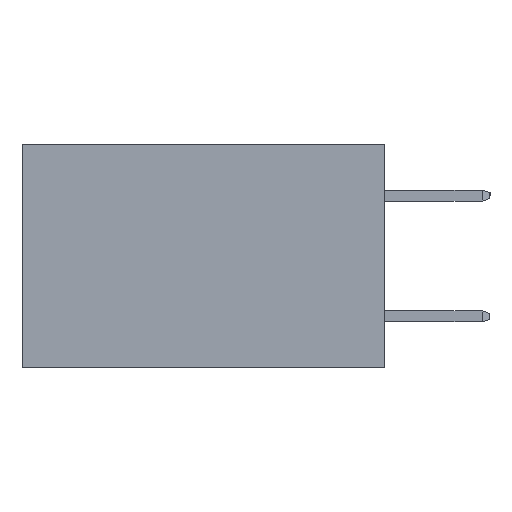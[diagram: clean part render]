
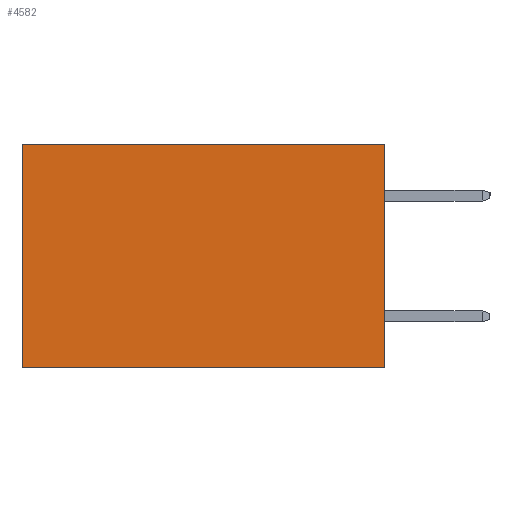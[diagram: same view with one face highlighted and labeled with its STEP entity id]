
A CAD part, left-side view. The second image highlights one B-rep face of the part: STEP entity #4582.
In plain terms, the highlighted planar face has unit normal (-1, 0, 0).
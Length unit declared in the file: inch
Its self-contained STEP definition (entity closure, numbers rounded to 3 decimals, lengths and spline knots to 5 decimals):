
#399 = EDGE_CURVE ( 'NONE', #7651, #2907, #5910, .T. ) ;
#801 = VECTOR ( 'NONE', #2639, 39.37008 ) ;
#963 = CARTESIAN_POINT ( 'NONE',  ( 0.2615, 0., -0.37 ) ) ;
#982 = VECTOR ( 'NONE', #10134, 39.37008 ) ;
#1044 = CARTESIAN_POINT ( 'NONE',  ( 0.2615, 0.6, 0. ) ) ;
#1580 = ORIENTED_EDGE ( 'NONE', *, *, #6989, .T. ) ;
#1996 = DIRECTION ( 'NONE',  ( 0., 0., -1. ) ) ;
#2310 = VECTOR ( 'NONE', #3495, 39.37008 ) ;
#2639 = DIRECTION ( 'NONE',  ( 0., 1., 0. ) ) ;
#2876 = LINE ( 'NONE', #9438, #4358 ) ;
#2907 = VERTEX_POINT ( 'NONE', #3697 ) ;
#3284 = AXIS2_PLACEMENT_3D ( 'NONE', #9940, #5931, #1996 ) ;
#3495 = DIRECTION ( 'NONE',  ( 0., 0., -1. ) ) ;
#3570 = CARTESIAN_POINT ( 'NONE',  ( 0.2615, 0.6, -0.37 ) ) ;
#3697 = CARTESIAN_POINT ( 'NONE',  ( 0.2615, 0.6, -0.37 ) ) ;
#4270 = ORIENTED_EDGE ( 'NONE', *, *, #8284, .F. ) ;
#4313 = PLANE ( 'NONE',  #3284 ) ;
#4358 = VECTOR ( 'NONE', #10282, 39.37008 ) ;
#4582 = ADVANCED_FACE ( 'NONE', ( #10095 ), #4313, .F. ) ;
#4598 = EDGE_LOOP ( 'NONE', ( #10310, #4270, #10232, #1580 ) ) ;
#5000 = VERTEX_POINT ( 'NONE', #9087 ) ;
#5237 = VERTEX_POINT ( 'NONE', #10238 ) ;
#5910 = LINE ( 'NONE', #3570, #982 ) ;
#5931 = DIRECTION ( 'NONE',  ( 1., 0., 0. ) ) ;
#6442 = EDGE_CURVE ( 'NONE', #5237, #5000, #9810, .T. ) ;
#6989 = EDGE_CURVE ( 'NONE', #5237, #7651, #8996, .T. ) ;
#7304 = CARTESIAN_POINT ( 'NONE',  ( 0.2615, 0., 0. ) ) ;
#7651 = VERTEX_POINT ( 'NONE', #1044 ) ;
#8284 = EDGE_CURVE ( 'NONE', #5000, #2907, #2876, .T. ) ;
#8996 = LINE ( 'NONE', #7304, #801 ) ;
#9087 = CARTESIAN_POINT ( 'NONE',  ( 0.2615, 0., -0.37 ) ) ;
#9438 = CARTESIAN_POINT ( 'NONE',  ( 0.2615, 0., -0.37 ) ) ;
#9810 = LINE ( 'NONE', #963, #2310 ) ;
#9940 = CARTESIAN_POINT ( 'NONE',  ( 0.2615, 0., -0.37 ) ) ;
#10095 = FACE_OUTER_BOUND ( 'NONE', #4598, .T. ) ;
#10134 = DIRECTION ( 'NONE',  ( 0., 0., -1. ) ) ;
#10232 = ORIENTED_EDGE ( 'NONE', *, *, #6442, .F. ) ;
#10238 = CARTESIAN_POINT ( 'NONE',  ( 0.2615, 0., 0. ) ) ;
#10282 = DIRECTION ( 'NONE',  ( 0., 1., 0. ) ) ;
#10310 = ORIENTED_EDGE ( 'NONE', *, *, #399, .T. ) ;
